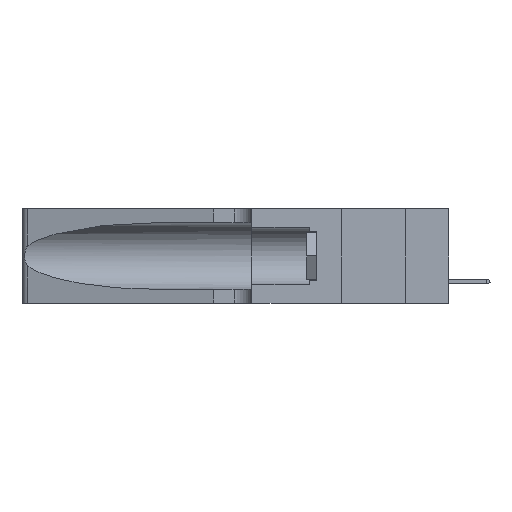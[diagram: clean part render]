
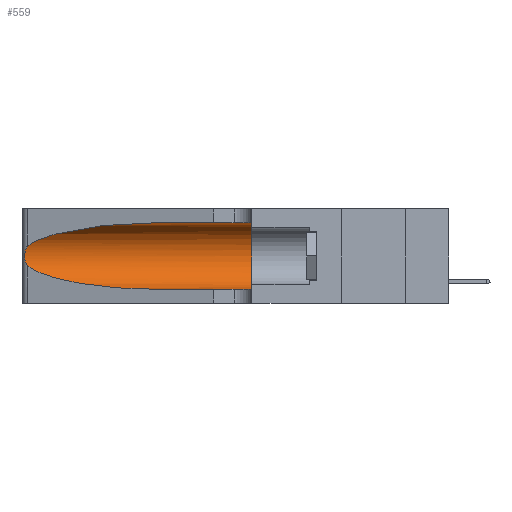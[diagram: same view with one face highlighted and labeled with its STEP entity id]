
A CAD part, left-side view. The second image highlights one B-rep face of the part: STEP entity #559.
In plain terms, the highlighted cylindrical face has radius 3.308 mm (diameter 6.617 mm), a partial arc.
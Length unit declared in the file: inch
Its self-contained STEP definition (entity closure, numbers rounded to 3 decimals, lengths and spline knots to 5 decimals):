
#114 = CARTESIAN_POINT ( 'NONE',  ( 0.25787, 1.23484, 0.2124 ) ) ;
#559 = ADVANCED_FACE ( 'NONE', ( #20277 ), #42116, .F. ) ;
#679 = CARTESIAN_POINT ( 'NONE',  ( 0.1305, 1.61858, 0.05475 ) ) ;
#1835 = CARTESIAN_POINT ( 'NONE',  ( 0.1305, 0.35, 0.185 ) ) ;
#3726 = CARTESIAN_POINT ( 'NONE',  ( 0.18966, 0.96281, 0.31525 ) ) ;
#3755 = CARTESIAN_POINT ( 'NONE',  ( 0.25487, 1.22718, 0.14631 ) ) ;
#4172 = EDGE_CURVE ( 'NONE', #48312, #4488, #48130, .T. ) ;
#4250 = VERTEX_POINT ( 'NONE', #31085 ) ;
#4488 = VERTEX_POINT ( 'NONE', #20644 ) ;
#4827 = ORIENTED_EDGE ( 'NONE', *, *, #4172, .T. ) ;
#7562 = CARTESIAN_POINT ( 'NONE',  ( 0.1305, 0.72297, 0.31525 ) ) ;
#7865 = CARTESIAN_POINT ( 'NONE',  ( 0.26075, 1.23896, 0.19203 ) ) ;
#8187 = CARTESIAN_POINT ( 'NONE',  ( 0.25856, 1.23593, 0.16098 ) ) ;
#8588 = DIRECTION ( 'NONE',  ( 0., -1., 0. ) ) ;
#9294 = VECTOR ( 'NONE', #25932, 39.37008 ) ;
#11180 = CARTESIAN_POINT ( 'NONE',  ( 0.25487, 1.22718, 0.14631 ) ) ;
#11355 = CARTESIAN_POINT ( 'NONE',  ( 0.25854, 1.2359, 0.20912 ) ) ;
#11819 = CARTESIAN_POINT ( 'NONE',  ( 0.26017, 1.23833, 0.17102 ) ) ;
#11970 = CARTESIAN_POINT ( 'NONE',  ( 0.25555, 1.22993, 0.14849 ) ) ;
#12080 = EDGE_CURVE ( 'NONE', #42541, #4250, #44486, .T. ) ;
#12552 = VERTEX_POINT ( 'NONE', #14539 ) ;
#14539 = CARTESIAN_POINT ( 'NONE',  ( 0.1305, 0.35, 0.05475 ) ) ;
#14675 = CARTESIAN_POINT ( 'NONE',  ( 0.1305, 1.61858, 0.31525 ) ) ;
#17023 = ORIENTED_EDGE ( 'NONE', *, *, #29120, .F. ) ;
#20087 = EDGE_LOOP ( 'NONE', ( #4827, #27268, #35758, #39524, #36787, #17023 ) ) ;
#20277 = FACE_OUTER_BOUND ( 'NONE', #20087, .T. ) ;
#20644 = CARTESIAN_POINT ( 'NONE',  ( 0.25487, 1.22718, 0.22369 ) ) ;
#21449 = CARTESIAN_POINT ( 'NONE',  ( 0.25487, 1.22718, 0.14631 ) ) ;
#21624 = CARTESIAN_POINT ( 'NONE',  ( 0.18966, 0.96281, 0.05475 ) ) ;
#21779 = VERTEX_POINT ( 'NONE', #43993 ) ;
#22994 = CARTESIAN_POINT ( 'NONE',  ( 0.25789, 1.23486, 0.15765 ) ) ;
#23229 = LINE ( 'NONE', #679, #24437 ) ;
#24437 = VECTOR ( 'NONE', #31318, 39.37008 ) ;
#25932 = DIRECTION ( 'NONE',  ( 0., -1., 0. ) ) ;
#26352 = LINE ( 'NONE', #14675, #9294 ) ;
#26522 = AXIS2_PLACEMENT_3D ( 'NONE', #1835, #28362, #32300 ) ;
#27268 = ORIENTED_EDGE ( 'NONE', *, *, #48238, .T. ) ;
#28362 = DIRECTION ( 'NONE',  ( 0., 1., 0. ) ) ;
#29120 = EDGE_CURVE ( 'NONE', #48312, #21779, #26352, .T. ) ;
#29168 = CARTESIAN_POINT ( 'NONE',  ( 0.1305, 0.72297, 0.05475 ) ) ;
#30406 = CARTESIAN_POINT ( 'NONE',  ( 0.26075, 1.23896, 0.178 ) ) ;
#31085 = CARTESIAN_POINT ( 'NONE',  ( 0.1305, 0.72297, 0.05475 ) ) ;
#31318 = DIRECTION ( 'NONE',  ( 0., -1., 0. ) ) ;
#32300 = DIRECTION ( 'NONE',  ( 0., 0., 1. ) ) ;
#32340 = EDGE_CURVE ( 'NONE', #21779, #12552, #35373, .T. ) ;
#34510 = CARTESIAN_POINT ( 'NONE',  ( 0.26018, 1.23835, 0.19895 ) ) ;
#35373 = CIRCLE ( 'NONE', #26522, 0.13025 ) ;
#35758 = ORIENTED_EDGE ( 'NONE', *, *, #12080, .T. ) ;
#36787 = ORIENTED_EDGE ( 'NONE', *, *, #32340, .F. ) ;
#37490 = CARTESIAN_POINT ( 'NONE',  ( 0.1305, 0.72297, 0.31525 ) ) ;
#39037 = DIRECTION ( 'NONE',  ( 0., 0., -1. ) ) ;
#39524 = ORIENTED_EDGE ( 'NONE', *, *, #46052, .T. ) ;
#41140 = CARTESIAN_POINT ( 'NONE',  ( 0.25555, 1.22994, 0.2215 ) ) ;
#41457 = CARTESIAN_POINT ( 'NONE',  ( 0.25639, 1.23184, 0.21858 ) ) ;
#42061 = CARTESIAN_POINT ( 'NONE',  ( 0.25639, 1.23186, 0.15144 ) ) ;
#42116 = CYLINDRICAL_SURFACE ( 'NONE', #48673, 0.13025 ) ;
#42541 = VERTEX_POINT ( 'NONE', #11180 ) ;
#42969 = CARTESIAN_POINT ( 'NONE',  ( 0.1305, 1.61858, 0.185 ) ) ;
#43356 = CARTESIAN_POINT ( 'NONE',  ( 0.25487, 1.22718, 0.22369 ) ) ;
#43993 = CARTESIAN_POINT ( 'NONE',  ( 0.1305, 0.35, 0.31525 ) ) ;
#44486 =( BOUNDED_CURVE ( )  B_SPLINE_CURVE ( 3, ( #21449, #47786, #21624, #29168 ),
 .UNSPECIFIED., .F., .F. ) 
 B_SPLINE_CURVE_WITH_KNOTS ( ( 4, 4 ),
 ( 3.44316, 4.71239 ),
 .UNSPECIFIED. ) 
 CURVE ( )  GEOMETRIC_REPRESENTATION_ITEM ( )  RATIONAL_B_SPLINE_CURVE ( ( 1., 0.87, 0.87, 1. ) ) 
 REPRESENTATION_ITEM ( '' )  );
#44769 = CARTESIAN_POINT ( 'NONE',  ( 0.25487, 1.22718, 0.22369 ) ) ;
#44773 = B_SPLINE_CURVE_WITH_KNOTS ( 'NONE', 3,
 ( #44769, #41140, #41457, #114, #11355, #34510, #7865, #30406, #11819, #8187, #22994, #42061, #11970, #3755 ),
 .UNSPECIFIED., .F., .F.,
 ( 4, 2, 2, 2, 2, 2, 4 ),
 ( 0., 0.00027, 0.00053, 0.00107, 0.0016, 0.00187, 0.00214 ),
 .UNSPECIFIED. ) ;
#45194 = CARTESIAN_POINT ( 'NONE',  ( 0.2373, 1.15595, 0.28018 ) ) ;
#46052 = EDGE_CURVE ( 'NONE', #4250, #12552, #23229, .T. ) ;
#47786 = CARTESIAN_POINT ( 'NONE',  ( 0.2373, 1.15595, 0.08982 ) ) ;
#48130 =( BOUNDED_CURVE ( )  B_SPLINE_CURVE ( 3, ( #37490, #3726, #45194, #43356 ),
 .UNSPECIFIED., .F., .T. ) 
 B_SPLINE_CURVE_WITH_KNOTS ( ( 4, 4 ),
 ( 1.5708, 2.84003 ),
 .UNSPECIFIED. ) 
 CURVE ( )  GEOMETRIC_REPRESENTATION_ITEM ( )  RATIONAL_B_SPLINE_CURVE ( ( 1., 0.87, 0.87, 1. ) ) 
 REPRESENTATION_ITEM ( '' )  );
#48238 = EDGE_CURVE ( 'NONE', #4488, #42541, #44773, .T. ) ;
#48312 = VERTEX_POINT ( 'NONE', #7562 ) ;
#48673 = AXIS2_PLACEMENT_3D ( 'NONE', #42969, #8588, #39037 ) ;
